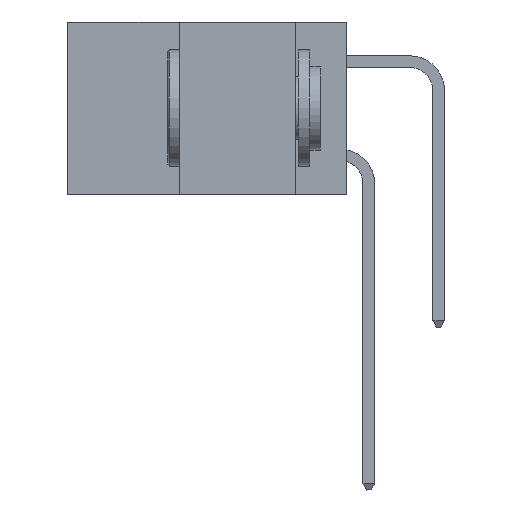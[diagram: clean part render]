
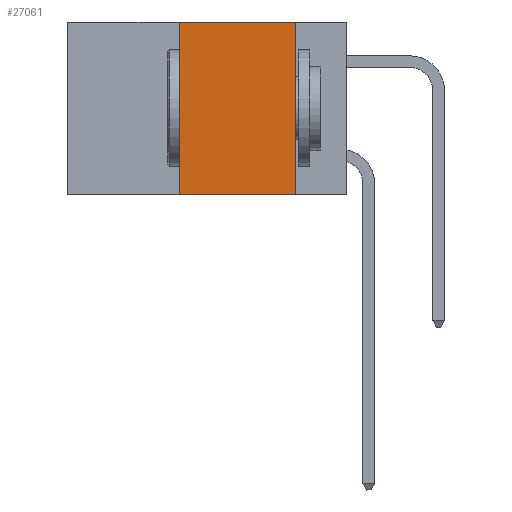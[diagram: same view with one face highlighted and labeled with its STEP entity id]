
A CAD part, left-side view. The second image highlights one B-rep face of the part: STEP entity #27061.
In plain terms, the highlighted planar face has unit normal (-1, 0, 0).
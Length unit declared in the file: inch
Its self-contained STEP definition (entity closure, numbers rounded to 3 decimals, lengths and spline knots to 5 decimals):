
#506 = FACE_OUTER_BOUND ( 'NONE', #11681, .T. ) ;
#819 = EDGE_CURVE ( 'NONE', #16147, #24828, #5247, .T. ) ;
#3524 = DIRECTION ( 'NONE',  ( 0., -1., 0. ) ) ;
#3686 = DIRECTION ( 'NONE',  ( 0., 0., 1. ) ) ;
#3758 = VECTOR ( 'NONE', #29450, 39.37008 ) ;
#4394 = VECTOR ( 'NONE', #3524, 39.37008 ) ;
#5247 = LINE ( 'NONE', #26866, #23471 ) ;
#5946 = CARTESIAN_POINT ( 'NONE',  ( 0., 0.36, -0.37 ) ) ;
#6160 = EDGE_CURVE ( 'NONE', #24828, #19055, #28493, .T. ) ;
#6727 = ORIENTED_EDGE ( 'NONE', *, *, #6955, .T. ) ;
#6955 = EDGE_CURVE ( 'NONE', #16147, #14533, #28814, .T. ) ;
#7467 = CARTESIAN_POINT ( 'NONE',  ( 0., 0.11, -0.37 ) ) ;
#8319 = CARTESIAN_POINT ( 'NONE',  ( 0., 0.11, 0. ) ) ;
#8753 = AXIS2_PLACEMENT_3D ( 'NONE', #20502, #22800, #17995 ) ;
#9285 = ORIENTED_EDGE ( 'NONE', *, *, #23773, .F. ) ;
#10588 = DIRECTION ( 'NONE',  ( 0., 0., -1. ) ) ;
#11102 = CARTESIAN_POINT ( 'NONE',  ( 0., 0.6, 0. ) ) ;
#11681 = EDGE_LOOP ( 'NONE', ( #9285, #13899, #18285, #6727 ) ) ;
#11873 = VECTOR ( 'NONE', #10588, 39.37008 ) ;
#13899 = ORIENTED_EDGE ( 'NONE', *, *, #6160, .F. ) ;
#14533 = VERTEX_POINT ( 'NONE', #7467 ) ;
#16147 = VERTEX_POINT ( 'NONE', #5946 ) ;
#17995 = DIRECTION ( 'NONE',  ( 0., 0., -1. ) ) ;
#18285 = ORIENTED_EDGE ( 'NONE', *, *, #819, .F. ) ;
#19055 = VERTEX_POINT ( 'NONE', #22850 ) ;
#20395 = PLANE ( 'NONE',  #8753 ) ;
#20502 = CARTESIAN_POINT ( 'NONE',  ( 0., 0.6, 0. ) ) ;
#22138 = CARTESIAN_POINT ( 'NONE',  ( 0., 0.6, -0.37 ) ) ;
#22800 = DIRECTION ( 'NONE',  ( 1., 0., 0. ) ) ;
#22850 = CARTESIAN_POINT ( 'NONE',  ( 0., 0.11, 0. ) ) ;
#23471 = VECTOR ( 'NONE', #3686, 39.37008 ) ;
#23773 = EDGE_CURVE ( 'NONE', #19055, #14533, #29772, .T. ) ;
#24828 = VERTEX_POINT ( 'NONE', #28962 ) ;
#26866 = CARTESIAN_POINT ( 'NONE',  ( 0., 0.36, 0. ) ) ;
#27061 = ADVANCED_FACE ( 'NONE', ( #506 ), #20395, .F. ) ;
#28493 = LINE ( 'NONE', #11102, #3758 ) ;
#28814 = LINE ( 'NONE', #22138, #4394 ) ;
#28962 = CARTESIAN_POINT ( 'NONE',  ( 0., 0.36, 0. ) ) ;
#29450 = DIRECTION ( 'NONE',  ( 0., -1., 0. ) ) ;
#29772 = LINE ( 'NONE', #8319, #11873 ) ;
